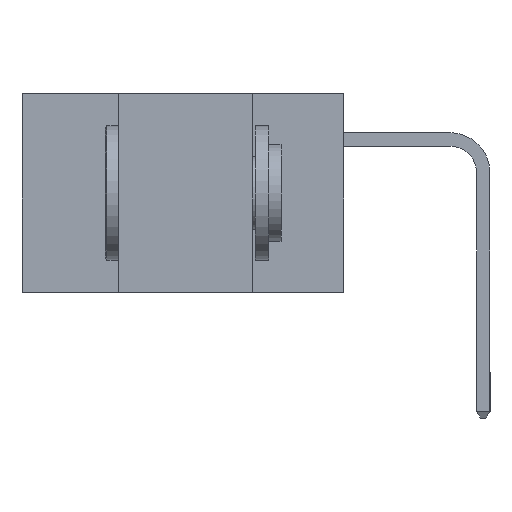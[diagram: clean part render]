
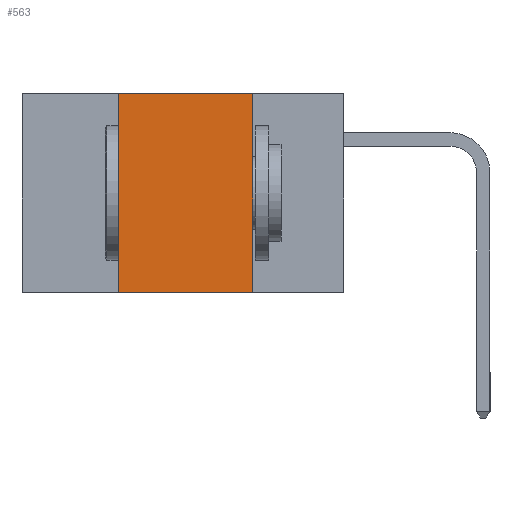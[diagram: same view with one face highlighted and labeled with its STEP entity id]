
A CAD part, left-side view. The second image highlights one B-rep face of the part: STEP entity #563.
In plain terms, the highlighted planar face has unit normal (-1, 0, 0).
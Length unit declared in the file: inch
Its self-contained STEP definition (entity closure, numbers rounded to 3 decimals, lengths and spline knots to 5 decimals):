
#394 = CARTESIAN_POINT ( 'NONE',  ( 0., 0.17, 0. ) ) ;
#434 = DIRECTION ( 'NONE',  ( 0., -1., 0. ) ) ;
#536 = ORIENTED_EDGE ( 'NONE', *, *, #5959, .F. ) ;
#563 = ADVANCED_FACE ( 'NONE', ( #8835 ), #14031, .F. ) ;
#1154 = EDGE_CURVE ( 'NONE', #1279, #4925, #2568, .T. ) ;
#1279 = VERTEX_POINT ( 'NONE', #7944 ) ;
#2122 = VERTEX_POINT ( 'NONE', #5556 ) ;
#2568 = LINE ( 'NONE', #4922, #14259 ) ;
#2622 = CARTESIAN_POINT ( 'NONE',  ( 0., 0.6, -0.37 ) ) ;
#3369 = ORIENTED_EDGE ( 'NONE', *, *, #7698, .T. ) ;
#3434 = VECTOR ( 'NONE', #5502, 39.37008 ) ;
#4324 = LINE ( 'NONE', #2622, #15413 ) ;
#4922 = CARTESIAN_POINT ( 'NONE',  ( 0., 0.42, 0. ) ) ;
#4925 = VERTEX_POINT ( 'NONE', #12668 ) ;
#4967 = DIRECTION ( 'NONE',  ( 1., 0., 0. ) ) ;
#5502 = DIRECTION ( 'NONE',  ( 0., 0., -1. ) ) ;
#5556 = CARTESIAN_POINT ( 'NONE',  ( 0., 0.17, -0.37 ) ) ;
#5959 = EDGE_CURVE ( 'NONE', #15296, #2122, #12051, .T. ) ;
#6241 = DIRECTION ( 'NONE',  ( 0., 0., -1. ) ) ;
#7468 = CARTESIAN_POINT ( 'NONE',  ( 0., 0.6, 0. ) ) ;
#7485 = LINE ( 'NONE', #11541, #14371 ) ;
#7698 = EDGE_CURVE ( 'NONE', #1279, #2122, #4324, .T. ) ;
#7944 = CARTESIAN_POINT ( 'NONE',  ( 0., 0.42, -0.37 ) ) ;
#8424 = EDGE_CURVE ( 'NONE', #4925, #15296, #7485, .T. ) ;
#8459 = ORIENTED_EDGE ( 'NONE', *, *, #1154, .F. ) ;
#8835 = FACE_OUTER_BOUND ( 'NONE', #10854, .T. ) ;
#9106 = DIRECTION ( 'NONE',  ( 0., -1., 0. ) ) ;
#10781 = CARTESIAN_POINT ( 'NONE',  ( 0., 0.17, 0. ) ) ;
#10854 = EDGE_LOOP ( 'NONE', ( #536, #15984, #8459, #3369 ) ) ;
#11373 = DIRECTION ( 'NONE',  ( 0., 0., 1. ) ) ;
#11541 = CARTESIAN_POINT ( 'NONE',  ( 0., 0.6, 0. ) ) ;
#12051 = LINE ( 'NONE', #10781, #3434 ) ;
#12105 = AXIS2_PLACEMENT_3D ( 'NONE', #7468, #4967, #6241 ) ;
#12668 = CARTESIAN_POINT ( 'NONE',  ( 0., 0.42, 0. ) ) ;
#14031 = PLANE ( 'NONE',  #12105 ) ;
#14259 = VECTOR ( 'NONE', #11373, 39.37008 ) ;
#14371 = VECTOR ( 'NONE', #9106, 39.37008 ) ;
#15296 = VERTEX_POINT ( 'NONE', #394 ) ;
#15413 = VECTOR ( 'NONE', #434, 39.37008 ) ;
#15984 = ORIENTED_EDGE ( 'NONE', *, *, #8424, .F. ) ;
